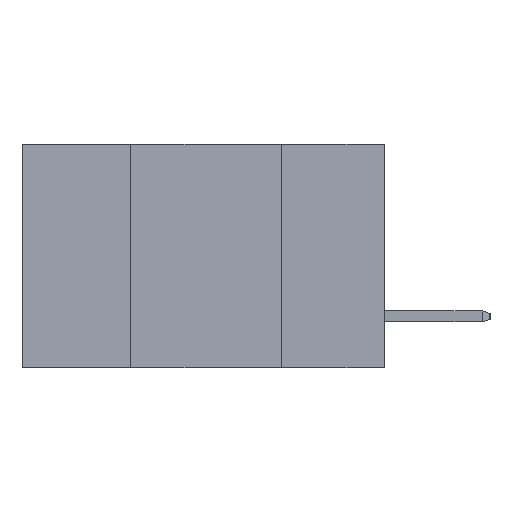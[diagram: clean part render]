
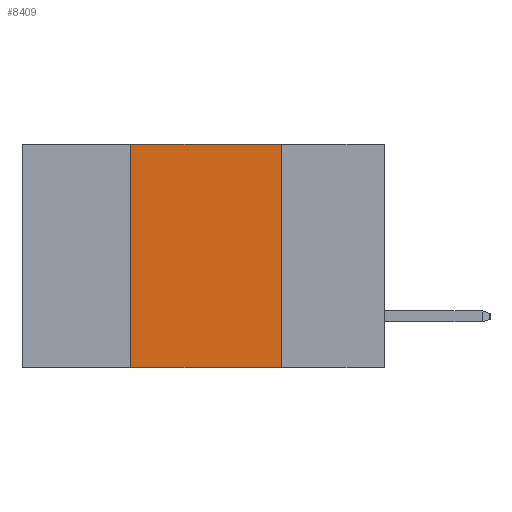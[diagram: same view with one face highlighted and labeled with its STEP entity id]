
A CAD part, left-side view. The second image highlights one B-rep face of the part: STEP entity #8409.
In plain terms, the highlighted planar face has unit normal (-1, 0, 0).
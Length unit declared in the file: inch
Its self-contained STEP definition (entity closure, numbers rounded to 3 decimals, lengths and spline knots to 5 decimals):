
#951 = VECTOR ( 'NONE', #3859, 39.37008 ) ;
#984 = VERTEX_POINT ( 'NONE', #7768 ) ;
#2642 = EDGE_LOOP ( 'NONE', ( #5768, #10934, #11751, #6091 ) ) ;
#3095 = VERTEX_POINT ( 'NONE', #4262 ) ;
#3171 = VECTOR ( 'NONE', #8177, 39.37008 ) ;
#3596 = CARTESIAN_POINT ( 'NONE',  ( 0., 0.17, -0.37 ) ) ;
#3629 = EDGE_CURVE ( 'NONE', #6077, #984, #6108, .T. ) ;
#3717 = LINE ( 'NONE', #3967, #951 ) ;
#3788 = EDGE_CURVE ( 'NONE', #7954, #3095, #4327, .T. ) ;
#3859 = DIRECTION ( 'NONE',  ( 0., -1., 0. ) ) ;
#3967 = CARTESIAN_POINT ( 'NONE',  ( 0., 0.6, -0.37 ) ) ;
#4199 = DIRECTION ( 'NONE',  ( 0., 0., -1. ) ) ;
#4262 = CARTESIAN_POINT ( 'NONE',  ( 0., 0.17, -0.37 ) ) ;
#4327 = LINE ( 'NONE', #3596, #6549 ) ;
#4335 = CARTESIAN_POINT ( 'NONE',  ( 0., 0.42, -0.37 ) ) ;
#4775 = PLANE ( 'NONE',  #4800 ) ;
#4800 = AXIS2_PLACEMENT_3D ( 'NONE', #12065, #11237, #5730 ) ;
#5726 = EDGE_CURVE ( 'NONE', #6077, #3095, #3717, .T. ) ;
#5730 = DIRECTION ( 'NONE',  ( 0., 0., -1. ) ) ;
#5768 = ORIENTED_EDGE ( 'NONE', *, *, #3788, .F. ) ;
#6077 = VERTEX_POINT ( 'NONE', #4335 ) ;
#6091 = ORIENTED_EDGE ( 'NONE', *, *, #5726, .T. ) ;
#6108 = LINE ( 'NONE', #11959, #8347 ) ;
#6128 = CARTESIAN_POINT ( 'NONE',  ( 0., 0.17, 0. ) ) ;
#6245 = CARTESIAN_POINT ( 'NONE',  ( 0., 0.6, 0. ) ) ;
#6549 = VECTOR ( 'NONE', #4199, 39.37008 ) ;
#7768 = CARTESIAN_POINT ( 'NONE',  ( 0., 0.42, 0. ) ) ;
#7954 = VERTEX_POINT ( 'NONE', #6128 ) ;
#8077 = EDGE_CURVE ( 'NONE', #984, #7954, #10614, .T. ) ;
#8177 = DIRECTION ( 'NONE',  ( 0., -1., 0. ) ) ;
#8347 = VECTOR ( 'NONE', #11780, 39.37008 ) ;
#8409 = ADVANCED_FACE ( 'NONE', ( #9344 ), #4775, .F. ) ;
#9344 = FACE_OUTER_BOUND ( 'NONE', #2642, .T. ) ;
#10614 = LINE ( 'NONE', #6245, #3171 ) ;
#10934 = ORIENTED_EDGE ( 'NONE', *, *, #8077, .F. ) ;
#11237 = DIRECTION ( 'NONE',  ( 1., 0., 0. ) ) ;
#11751 = ORIENTED_EDGE ( 'NONE', *, *, #3629, .F. ) ;
#11780 = DIRECTION ( 'NONE',  ( 0., 0., 1. ) ) ;
#11959 = CARTESIAN_POINT ( 'NONE',  ( 0., 0.42, -0.37 ) ) ;
#12065 = CARTESIAN_POINT ( 'NONE',  ( 0., 0.6, 0. ) ) ;
